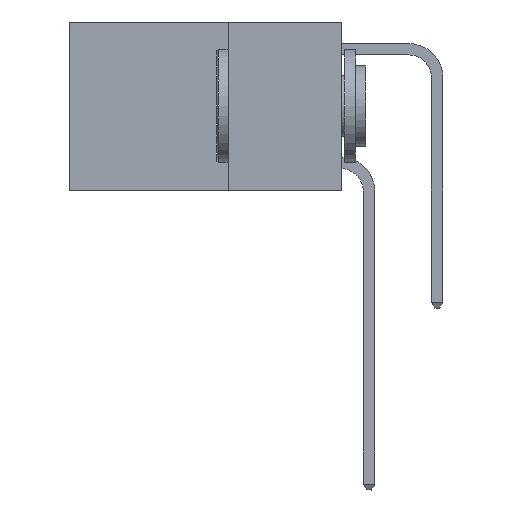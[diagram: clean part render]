
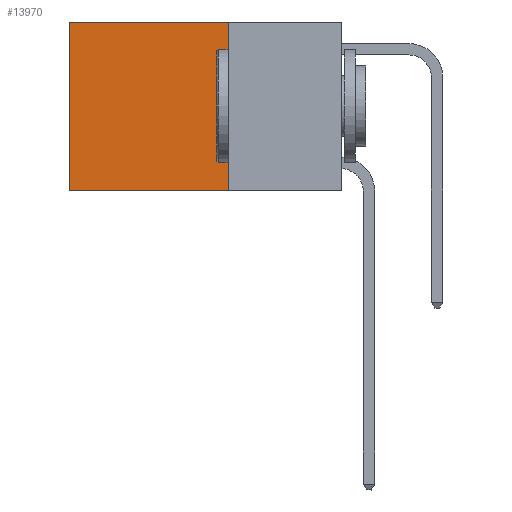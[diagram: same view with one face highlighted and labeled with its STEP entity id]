
A CAD part, left-side view. The second image highlights one B-rep face of the part: STEP entity #13970.
In plain terms, the highlighted planar face has unit normal (-1, 0, 0).
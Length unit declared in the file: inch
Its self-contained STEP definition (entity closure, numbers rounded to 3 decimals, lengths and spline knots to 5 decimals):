
#1054 = CARTESIAN_POINT ( 'NONE',  ( 0.2625, 0.25, -0.37 ) ) ;
#2709 = ORIENTED_EDGE ( 'NONE', *, *, #9672, .T. ) ;
#2991 = ORIENTED_EDGE ( 'NONE', *, *, #13316, .F. ) ;
#3165 = LINE ( 'NONE', #6564, #13888 ) ;
#3279 = CARTESIAN_POINT ( 'NONE',  ( 0.2625, 0.25, -0.37 ) ) ;
#3882 = LINE ( 'NONE', #1054, #20227 ) ;
#3963 = AXIS2_PLACEMENT_3D ( 'NONE', #8469, #6580, #11911 ) ;
#4285 = VERTEX_POINT ( 'NONE', #9964 ) ;
#4646 = LINE ( 'NONE', #4888, #10275 ) ;
#4888 = CARTESIAN_POINT ( 'NONE',  ( 0.2625, 0.6, 0. ) ) ;
#5014 = DIRECTION ( 'NONE',  ( 0., 0., -1. ) ) ;
#6015 = VERTEX_POINT ( 'NONE', #10219 ) ;
#6496 = EDGE_LOOP ( 'NONE', ( #2709, #2991, #8902, #18364 ) ) ;
#6564 = CARTESIAN_POINT ( 'NONE',  ( 0.2625, 0.25, 0. ) ) ;
#6580 = DIRECTION ( 'NONE',  ( 1., 0., 0. ) ) ;
#6986 = CARTESIAN_POINT ( 'NONE',  ( 0.2625, 0.6, 0. ) ) ;
#8009 = VERTEX_POINT ( 'NONE', #3279 ) ;
#8077 = LINE ( 'NONE', #9544, #12123 ) ;
#8469 = CARTESIAN_POINT ( 'NONE',  ( 0.2625, 0.25, 0. ) ) ;
#8902 = ORIENTED_EDGE ( 'NONE', *, *, #17857, .F. ) ;
#9544 = CARTESIAN_POINT ( 'NONE',  ( 0.2625, 0.25, 0. ) ) ;
#9672 = EDGE_CURVE ( 'NONE', #10914, #6015, #4646, .T. ) ;
#9964 = CARTESIAN_POINT ( 'NONE',  ( 0.2625, 0.25, 0. ) ) ;
#10057 = DIRECTION ( 'NONE',  ( 0., 0., -1. ) ) ;
#10219 = CARTESIAN_POINT ( 'NONE',  ( 0.2625, 0.6, -0.37 ) ) ;
#10275 = VECTOR ( 'NONE', #10057, 39.37008 ) ;
#10914 = VERTEX_POINT ( 'NONE', #6986 ) ;
#11343 = DIRECTION ( 'NONE',  ( 0., 1., 0. ) ) ;
#11911 = DIRECTION ( 'NONE',  ( 0., 0., -1. ) ) ;
#12123 = VECTOR ( 'NONE', #11343, 39.37008 ) ;
#13008 = DIRECTION ( 'NONE',  ( 0., 1., 0. ) ) ;
#13316 = EDGE_CURVE ( 'NONE', #8009, #6015, #3882, .T. ) ;
#13888 = VECTOR ( 'NONE', #5014, 39.37008 ) ;
#13970 = ADVANCED_FACE ( 'NONE', ( #21565 ), #21943, .F. ) ;
#14990 = EDGE_CURVE ( 'NONE', #4285, #10914, #8077, .T. ) ;
#17857 = EDGE_CURVE ( 'NONE', #4285, #8009, #3165, .T. ) ;
#18364 = ORIENTED_EDGE ( 'NONE', *, *, #14990, .T. ) ;
#20227 = VECTOR ( 'NONE', #13008, 39.37008 ) ;
#21565 = FACE_OUTER_BOUND ( 'NONE', #6496, .T. ) ;
#21943 = PLANE ( 'NONE',  #3963 ) ;
